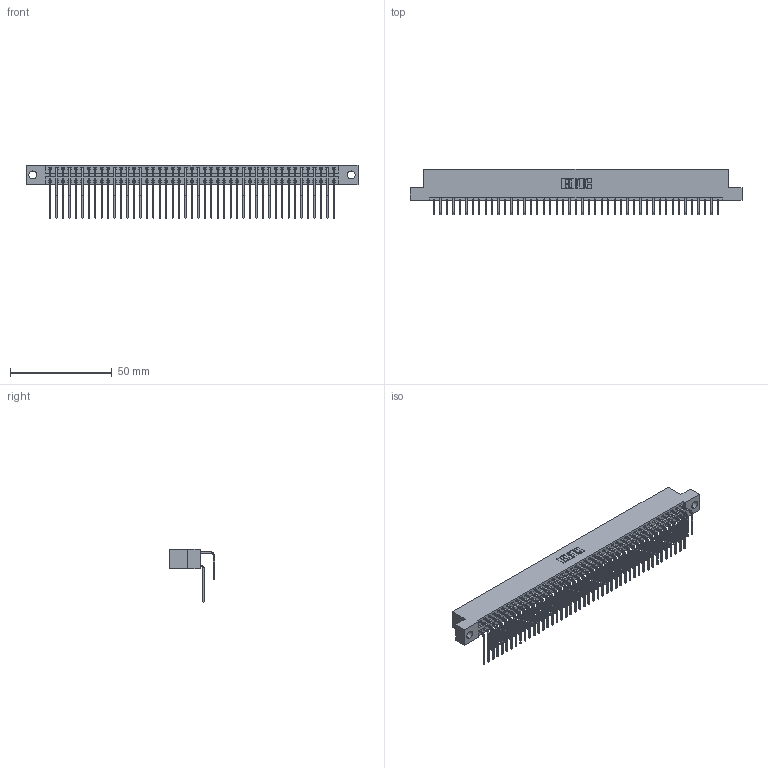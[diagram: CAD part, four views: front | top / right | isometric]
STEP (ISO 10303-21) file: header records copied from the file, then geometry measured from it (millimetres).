
FILE_DESCRIPTION (( 'STEP AP203' ), '1' );
FILE_NAME ('346-090-558-204.STEP', '2022-05-26T05:01:34', ( '' ), ( '' ), 'SwSTEP 2.0', 'SolidWorks 2020', '' );
FILE_SCHEMA (( 'CONFIG_CONTROL_DESIGN' ));
Length unit declared in the file: inch
Products named in the file (4): 345-292-001_558 Tail - 2; 345-292-001_558 559 Tail - 1; 346-090-558-204; 346 Part_Flush Mounting Lugs - 0.156 Dia-TH
Assembly tree (91 placements, depth 2):
  346-090-558-204
    346 Part_Flush Mounting Lugs - 0.156 Dia-TH
    345-292-001_558 559 Tail - 1  x45
    345-292-001_558 Tail - 2  x45
Bounding box: 163.45 x 22.16 x 26.16 mm (x, y, z)
Volume: 16374.8 mm3; surface area: 24894.1 mm2
Topology: 91 solids, 91 shells, 4996 faces, 14855 edges, 9782 vertices
Faces by surface type: plane 3420, cylinder 1576
Entity records: 31167 total; most frequent: CARTESIAN_POINT 5189, ORIENTED_EDGE 5070, DIRECTION 4595, EDGE_CURVE 2535, VECTOR 2183, LINE 2183, VERTEX_POINT 1686, AXIS2_PLACEMENT_3D 1206
